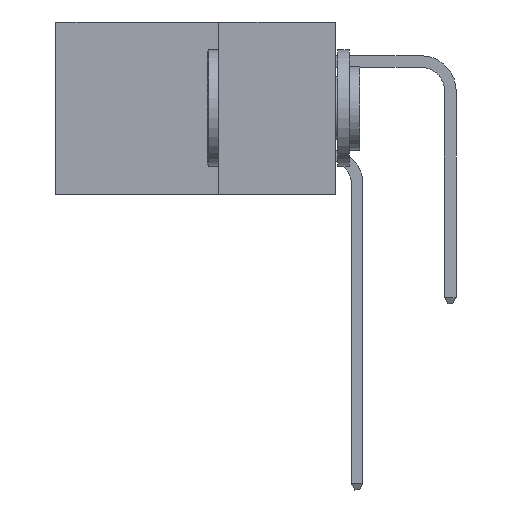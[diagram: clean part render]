
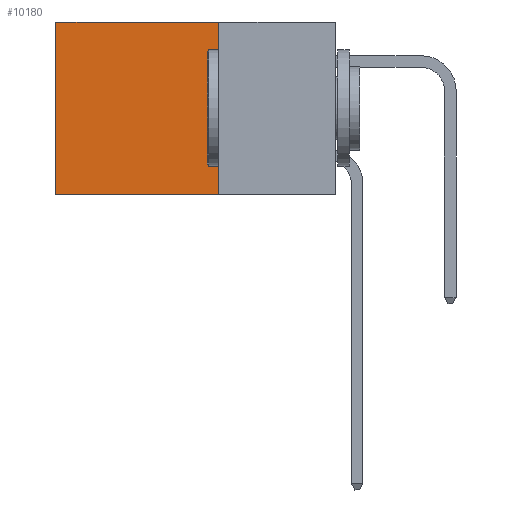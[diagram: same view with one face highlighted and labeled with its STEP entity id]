
A CAD part, left-side view. The second image highlights one B-rep face of the part: STEP entity #10180.
In plain terms, the highlighted planar face has unit normal (-1, 0, 0).
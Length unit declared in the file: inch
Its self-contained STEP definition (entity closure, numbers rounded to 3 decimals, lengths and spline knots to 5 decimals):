
#164 = VECTOR ( 'NONE', #8117, 39.37008 ) ;
#1003 = VERTEX_POINT ( 'NONE', #10533 ) ;
#1574 = DIRECTION ( 'NONE',  ( 0., 1., 0. ) ) ;
#1771 = CARTESIAN_POINT ( 'NONE',  ( 0.2875, 0.25, 0. ) ) ;
#2339 = DIRECTION ( 'NONE',  ( 0., 0., -1. ) ) ;
#3298 = CARTESIAN_POINT ( 'NONE',  ( 0.2875, 0.6, 0. ) ) ;
#4633 = VECTOR ( 'NONE', #1574, 39.37008 ) ;
#4650 = ORIENTED_EDGE ( 'NONE', *, *, #11464, .T. ) ;
#4925 = VECTOR ( 'NONE', #20519, 39.37008 ) ;
#5034 = EDGE_CURVE ( 'NONE', #28206, #16808, #15247, .T. ) ;
#6041 = ORIENTED_EDGE ( 'NONE', *, *, #27496, .T. ) ;
#8117 = DIRECTION ( 'NONE',  ( 0., 0., -1. ) ) ;
#9164 = ORIENTED_EDGE ( 'NONE', *, *, #23553, .F. ) ;
#9415 = DIRECTION ( 'NONE',  ( 0., 1., 0. ) ) ;
#10180 = ADVANCED_FACE ( 'NONE', ( #10964 ), #25836, .F. ) ;
#10533 = CARTESIAN_POINT ( 'NONE',  ( 0.2875, 0.6, -0.37 ) ) ;
#10535 = LINE ( 'NONE', #1771, #4633 ) ;
#10964 = FACE_OUTER_BOUND ( 'NONE', #20355, .T. ) ;
#11464 = EDGE_CURVE ( 'NONE', #17420, #1003, #28737, .T. ) ;
#11589 = DIRECTION ( 'NONE',  ( 1., 0., 0. ) ) ;
#11811 = AXIS2_PLACEMENT_3D ( 'NONE', #30717, #11589, #2339 ) ;
#15247 = LINE ( 'NONE', #17935, #4925 ) ;
#16581 = CARTESIAN_POINT ( 'NONE',  ( 0.2875, 0.6, 0. ) ) ;
#16630 = LINE ( 'NONE', #21214, #24474 ) ;
#16808 = VERTEX_POINT ( 'NONE', #29623 ) ;
#17420 = VERTEX_POINT ( 'NONE', #16581 ) ;
#17935 = CARTESIAN_POINT ( 'NONE',  ( 0.2875, 0.25, 0. ) ) ;
#20355 = EDGE_LOOP ( 'NONE', ( #4650, #9164, #22428, #6041 ) ) ;
#20519 = DIRECTION ( 'NONE',  ( 0., 0., -1. ) ) ;
#21214 = CARTESIAN_POINT ( 'NONE',  ( 0.2875, 0.25, -0.37 ) ) ;
#22428 = ORIENTED_EDGE ( 'NONE', *, *, #5034, .F. ) ;
#23553 = EDGE_CURVE ( 'NONE', #16808, #1003, #16630, .T. ) ;
#24474 = VECTOR ( 'NONE', #9415, 39.37008 ) ;
#25836 = PLANE ( 'NONE',  #11811 ) ;
#27496 = EDGE_CURVE ( 'NONE', #28206, #17420, #10535, .T. ) ;
#27583 = CARTESIAN_POINT ( 'NONE',  ( 0.2875, 0.25, 0. ) ) ;
#28206 = VERTEX_POINT ( 'NONE', #27583 ) ;
#28737 = LINE ( 'NONE', #3298, #164 ) ;
#29623 = CARTESIAN_POINT ( 'NONE',  ( 0.2875, 0.25, -0.37 ) ) ;
#30717 = CARTESIAN_POINT ( 'NONE',  ( 0.2875, 0.25, 0. ) ) ;
